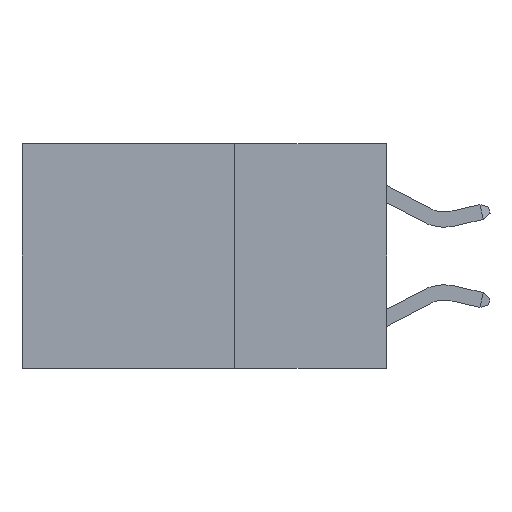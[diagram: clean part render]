
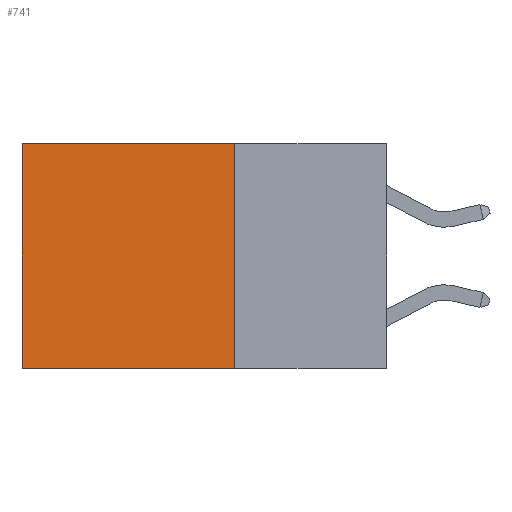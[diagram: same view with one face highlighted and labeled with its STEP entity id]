
A CAD part, left-side view. The second image highlights one B-rep face of the part: STEP entity #741.
In plain terms, the highlighted planar face has unit normal (-1, 0, 0).
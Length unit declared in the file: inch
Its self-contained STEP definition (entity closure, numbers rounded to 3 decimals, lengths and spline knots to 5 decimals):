
#12 = VECTOR ( 'NONE', #8509, 39.37008 ) ;
#128 = VECTOR ( 'NONE', #9734, 39.37008 ) ;
#741 = ADVANCED_FACE ( 'NONE', ( #6679 ), #4334, .F. ) ;
#769 = ORIENTED_EDGE ( 'NONE', *, *, #8512, .T. ) ;
#1349 = DIRECTION ( 'NONE',  ( 1., 0., 0. ) ) ;
#1646 = VECTOR ( 'NONE', #2609, 39.37008 ) ;
#1803 = ORIENTED_EDGE ( 'NONE', *, *, #2956, .T. ) ;
#2609 = DIRECTION ( 'NONE',  ( 0., 1., 0. ) ) ;
#2758 = LINE ( 'NONE', #8925, #1646 ) ;
#2956 = EDGE_CURVE ( 'NONE', #6354, #4019, #6628, .T. ) ;
#3614 = CARTESIAN_POINT ( 'NONE',  ( 0.2625, 0.25, 0. ) ) ;
#3769 = CARTESIAN_POINT ( 'NONE',  ( 0.2625, 0.25, 0. ) ) ;
#4019 = VERTEX_POINT ( 'NONE', #7784 ) ;
#4099 = CARTESIAN_POINT ( 'NONE',  ( 0.2625, 0.25, 0. ) ) ;
#4334 = PLANE ( 'NONE',  #6718 ) ;
#4582 = VECTOR ( 'NONE', #5416, 39.37008 ) ;
#4811 = LINE ( 'NONE', #5531, #12 ) ;
#5364 = VERTEX_POINT ( 'NONE', #9043 ) ;
#5416 = DIRECTION ( 'NONE',  ( 0., 0., -1. ) ) ;
#5531 = CARTESIAN_POINT ( 'NONE',  ( 0.2625, 0.6, 0. ) ) ;
#5631 = EDGE_CURVE ( 'NONE', #5364, #7858, #2758, .T. ) ;
#6332 = ORIENTED_EDGE ( 'NONE', *, *, #5631, .F. ) ;
#6354 = VERTEX_POINT ( 'NONE', #4099 ) ;
#6628 = LINE ( 'NONE', #3769, #128 ) ;
#6679 = FACE_OUTER_BOUND ( 'NONE', #8145, .T. ) ;
#6718 = AXIS2_PLACEMENT_3D ( 'NONE', #3614, #1349, #7587 ) ;
#7189 = EDGE_CURVE ( 'NONE', #6354, #5364, #9080, .T. ) ;
#7587 = DIRECTION ( 'NONE',  ( 0., 0., -1. ) ) ;
#7743 = ORIENTED_EDGE ( 'NONE', *, *, #7189, .F. ) ;
#7784 = CARTESIAN_POINT ( 'NONE',  ( 0.2625, 0.6, 0. ) ) ;
#7858 = VERTEX_POINT ( 'NONE', #9882 ) ;
#8145 = EDGE_LOOP ( 'NONE', ( #769, #6332, #7743, #1803 ) ) ;
#8509 = DIRECTION ( 'NONE',  ( 0., 0., -1. ) ) ;
#8512 = EDGE_CURVE ( 'NONE', #4019, #7858, #4811, .T. ) ;
#8925 = CARTESIAN_POINT ( 'NONE',  ( 0.2625, 0.25, -0.37 ) ) ;
#9031 = CARTESIAN_POINT ( 'NONE',  ( 0.2625, 0.25, 0. ) ) ;
#9043 = CARTESIAN_POINT ( 'NONE',  ( 0.2625, 0.25, -0.37 ) ) ;
#9080 = LINE ( 'NONE', #9031, #4582 ) ;
#9734 = DIRECTION ( 'NONE',  ( 0., 1., 0. ) ) ;
#9882 = CARTESIAN_POINT ( 'NONE',  ( 0.2625, 0.6, -0.37 ) ) ;
